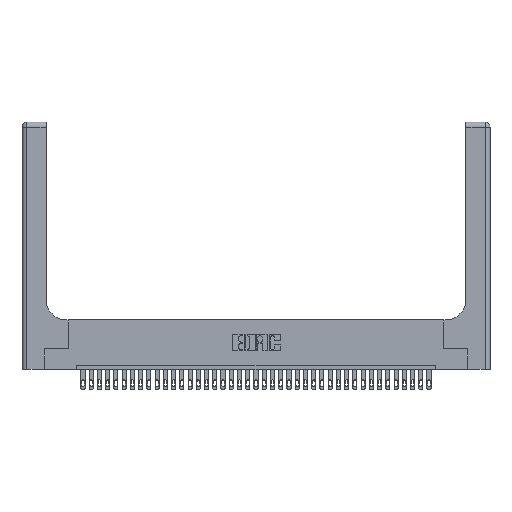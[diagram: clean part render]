
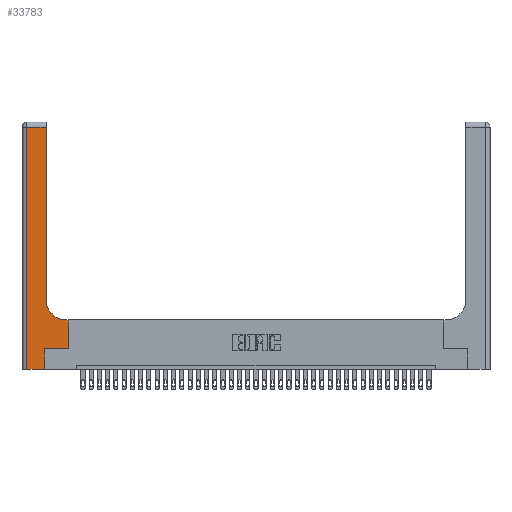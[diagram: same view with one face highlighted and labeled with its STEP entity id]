
A CAD part, top view. The second image highlights one B-rep face of the part: STEP entity #33783.
In plain terms, the highlighted planar face has unit normal (0, 0, 1).
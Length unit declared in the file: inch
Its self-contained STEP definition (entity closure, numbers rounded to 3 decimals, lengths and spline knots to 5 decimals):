
#64 = CARTESIAN_POINT ( 'NONE',  ( 0.06, 3., 0.37 ) ) ;
#549 = LINE ( 'NONE', #7881, #13194 ) ;
#1923 = VECTOR ( 'NONE', #26457, 39.37008 ) ;
#1991 = VECTOR ( 'NONE', #31264, 39.37008 ) ;
#2470 = CARTESIAN_POINT ( 'NONE',  ( 0.2915, 3., 0.37 ) ) ;
#3517 = ORIENTED_EDGE ( 'NONE', *, *, #28059, .T. ) ;
#4165 = CARTESIAN_POINT ( 'NONE',  ( 0.269, 0.25, 0.37 ) ) ;
#4673 = ORIENTED_EDGE ( 'NONE', *, *, #10269, .T. ) ;
#5236 = DIRECTION ( 'NONE',  ( 0., 1., 0. ) ) ;
#5411 = DIRECTION ( 'NONE',  ( -1., 0., 0. ) ) ;
#5511 = CARTESIAN_POINT ( 'NONE',  ( 0.5585, 0.6, 0.37 ) ) ;
#6971 = EDGE_CURVE ( 'NONE', #29425, #21383, #16153, .T. ) ;
#7026 = EDGE_LOOP ( 'NONE', ( #31357, #11025, #19692, #3517, #4673, #14161, #14025, #36615, #11037 ) ) ;
#7613 = VERTEX_POINT ( 'NONE', #26209 ) ;
#7881 = CARTESIAN_POINT ( 'NONE',  ( 0.5585, 0.25, 0.37 ) ) ;
#8084 = VECTOR ( 'NONE', #10707, 39.37008 ) ;
#8441 = CARTESIAN_POINT ( 'NONE',  ( 0.2915, 0.85, 0.37 ) ) ;
#9551 = VERTEX_POINT ( 'NONE', #12622 ) ;
#10098 = VERTEX_POINT ( 'NONE', #14204 ) ;
#10269 = EDGE_CURVE ( 'NONE', #9551, #31100, #19155, .T. ) ;
#10562 = VERTEX_POINT ( 'NONE', #12269 ) ;
#10707 = DIRECTION ( 'NONE',  ( -1., 0., 0. ) ) ;
#10775 = DIRECTION ( 'NONE',  ( 0., 1., 0. ) ) ;
#11025 = ORIENTED_EDGE ( 'NONE', *, *, #6971, .T. ) ;
#11037 = ORIENTED_EDGE ( 'NONE', *, *, #20542, .T. ) ;
#11264 = DIRECTION ( 'NONE',  ( 0., 1., 0. ) ) ;
#11616 = CARTESIAN_POINT ( 'NONE',  ( 0.06, 2.94, 0.37 ) ) ;
#12144 = AXIS2_PLACEMENT_3D ( 'NONE', #30716, #13570, #16700 ) ;
#12269 = CARTESIAN_POINT ( 'NONE',  ( 0.06, 0., 0.37 ) ) ;
#12622 = CARTESIAN_POINT ( 'NONE',  ( 0.269, 0., 0.37 ) ) ;
#12646 = LINE ( 'NONE', #34164, #33907 ) ;
#13194 = VECTOR ( 'NONE', #5236, 39.37008 ) ;
#13257 = VECTOR ( 'NONE', #10775, 39.37008 ) ;
#13410 = CARTESIAN_POINT ( 'NONE',  ( 0., 2.94, 0.37 ) ) ;
#13570 = DIRECTION ( 'NONE',  ( 0., 0., -1. ) ) ;
#14025 = ORIENTED_EDGE ( 'NONE', *, *, #34447, .T. ) ;
#14161 = ORIENTED_EDGE ( 'NONE', *, *, #20598, .T. ) ;
#14204 = CARTESIAN_POINT ( 'NONE',  ( 0.5415, 0.6, 0.37 ) ) ;
#14747 = DIRECTION ( 'NONE',  ( 0., -1., 0. ) ) ;
#16153 = LINE ( 'NONE', #13410, #8084 ) ;
#16198 = PLANE ( 'NONE',  #12144 ) ;
#16700 = DIRECTION ( 'NONE',  ( -1., 0., 0. ) ) ;
#17326 = VECTOR ( 'NONE', #11264, 39.37008 ) ;
#17984 = VECTOR ( 'NONE', #14747, 39.37008 ) ;
#19051 = LINE ( 'NONE', #22410, #1991 ) ;
#19155 = LINE ( 'NONE', #37122, #17326 ) ;
#19692 = ORIENTED_EDGE ( 'NONE', *, *, #30176, .T. ) ;
#20049 = VERTEX_POINT ( 'NONE', #8441 ) ;
#20542 = EDGE_CURVE ( 'NONE', #10098, #20049, #24377, .T. ) ;
#20598 = EDGE_CURVE ( 'NONE', #31100, #7613, #30268, .T. ) ;
#20867 = LINE ( 'NONE', #2470, #13257 ) ;
#21226 = AXIS2_PLACEMENT_3D ( 'NONE', #29537, #29788, #21307 ) ;
#21307 = DIRECTION ( 'NONE',  ( 1., 0., 0. ) ) ;
#21383 = VERTEX_POINT ( 'NONE', #11616 ) ;
#21552 = EDGE_CURVE ( 'NONE', #32403, #10098, #12646, .T. ) ;
#21632 = LINE ( 'NONE', #64, #17984 ) ;
#22410 = CARTESIAN_POINT ( 'NONE',  ( 0., 0., 0.37 ) ) ;
#24047 = FACE_OUTER_BOUND ( 'NONE', #7026, .T. ) ;
#24377 = CIRCLE ( 'NONE', #21226, 0.25 ) ;
#26209 = CARTESIAN_POINT ( 'NONE',  ( 0.5585, 0.25, 0.37 ) ) ;
#26457 = DIRECTION ( 'NONE',  ( 1., 0., 0. ) ) ;
#27434 = EDGE_CURVE ( 'NONE', #20049, #29425, #20867, .T. ) ;
#28059 = EDGE_CURVE ( 'NONE', #10562, #9551, #19051, .T. ) ;
#29425 = VERTEX_POINT ( 'NONE', #31123 ) ;
#29537 = CARTESIAN_POINT ( 'NONE',  ( 0.5415, 0.85, 0.37 ) ) ;
#29788 = DIRECTION ( 'NONE',  ( 0., 0., -1. ) ) ;
#30176 = EDGE_CURVE ( 'NONE', #21383, #10562, #21632, .T. ) ;
#30268 = LINE ( 'NONE', #36267, #1923 ) ;
#30716 = CARTESIAN_POINT ( 'NONE',  ( 0., 3., 0.37 ) ) ;
#31100 = VERTEX_POINT ( 'NONE', #4165 ) ;
#31123 = CARTESIAN_POINT ( 'NONE',  ( 0.2915, 2.94, 0.37 ) ) ;
#31264 = DIRECTION ( 'NONE',  ( 1., 0., 0. ) ) ;
#31357 = ORIENTED_EDGE ( 'NONE', *, *, #27434, .T. ) ;
#32403 = VERTEX_POINT ( 'NONE', #5511 ) ;
#33783 = ADVANCED_FACE ( 'NONE', ( #24047 ), #16198, .F. ) ;
#33907 = VECTOR ( 'NONE', #5411, 39.37008 ) ;
#34164 = CARTESIAN_POINT ( 'NONE',  ( 0.2915, 0.6, 0.37 ) ) ;
#34447 = EDGE_CURVE ( 'NONE', #7613, #32403, #549, .T. ) ;
#36267 = CARTESIAN_POINT ( 'NONE',  ( 0.269, 0.25, 0.37 ) ) ;
#36615 = ORIENTED_EDGE ( 'NONE', *, *, #21552, .T. ) ;
#37122 = CARTESIAN_POINT ( 'NONE',  ( 0.269, 0., 0.37 ) ) ;
